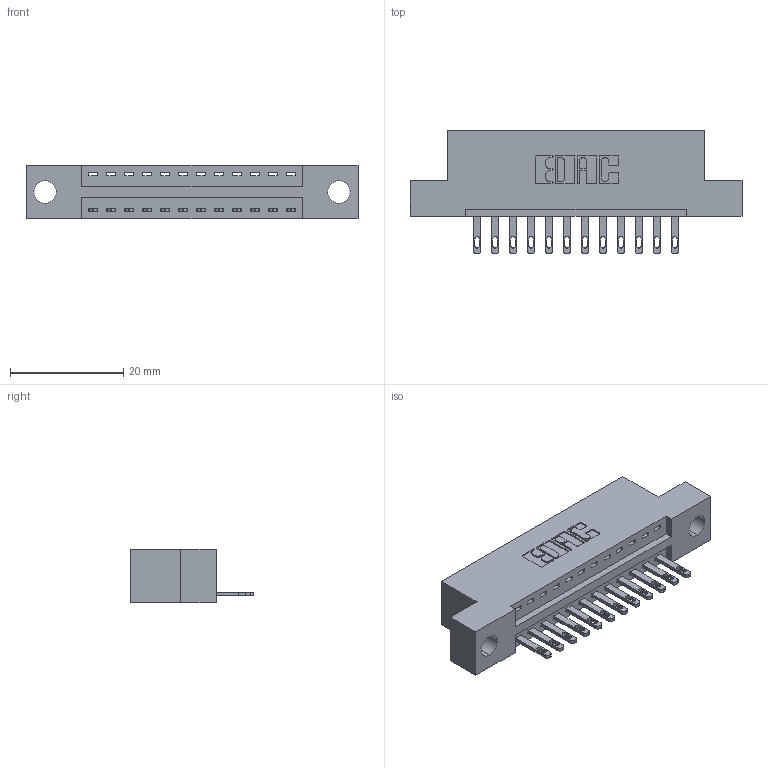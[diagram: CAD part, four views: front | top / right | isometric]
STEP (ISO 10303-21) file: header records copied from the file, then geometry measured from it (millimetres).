
FILE_DESCRIPTION (( 'STEP AP203' ), '1' );
FILE_NAME ('346-012-500-104.STEP', '2022-05-05T02:06:51', ( '' ), ( '' ), 'SwSTEP 2.0', 'SolidWorks 2020', '' );
FILE_SCHEMA (( 'CONFIG_CONTROL_DESIGN' ));
Length unit declared in the file: inch
Products named in the file (3): 346 Part_Flush Mounting Lugs - 0.156 Dia-TH; 346-012-500-104; 345-292-001_345-293-100
Assembly tree (13 placements, depth 2):
  346-012-500-104
    346 Part_Flush Mounting Lugs - 0.156 Dia-TH
    345-292-001_345-293-100  x12
Bounding box: 58.67 x 21.84 x 9.4 mm (x, y, z)
Volume: 5311.2 mm3; surface area: 6179.8 mm2
Topology: 13 solids, 13 shells, 784 faces, 2381 edges, 1586 vertices
Faces by surface type: plane 498, cylinder 286
Entity records: 11835 total; most frequent: CARTESIAN_POINT 2046, ORIENTED_EDGE 1990, DIRECTION 1843, EDGE_CURVE 995, VECTOR 811, LINE 811, VERTEX_POINT 662, AXIS2_PLACEMENT_3D 516
